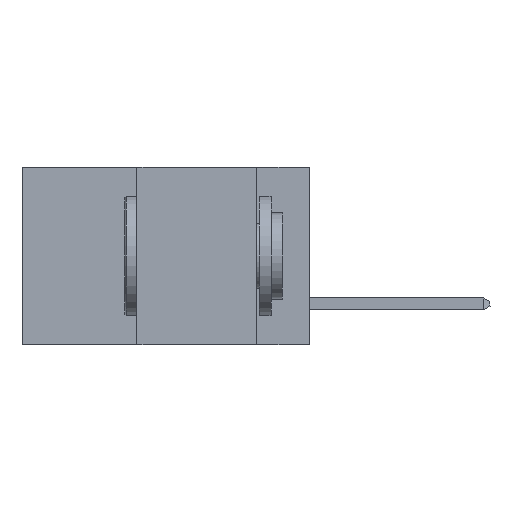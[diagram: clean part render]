
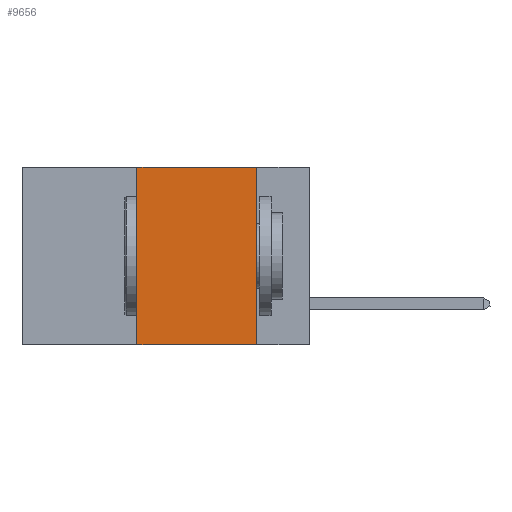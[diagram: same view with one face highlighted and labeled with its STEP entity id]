
A CAD part, left-side view. The second image highlights one B-rep face of the part: STEP entity #9656.
In plain terms, the highlighted planar face has unit normal (-1, 0, 0).
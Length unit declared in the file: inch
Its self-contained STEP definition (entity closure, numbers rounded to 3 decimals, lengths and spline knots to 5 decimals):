
#325 = EDGE_CURVE ( 'NONE', #12321, #18947, #13030, .T. ) ;
#816 = LINE ( 'NONE', #14119, #26722 ) ;
#1361 = CARTESIAN_POINT ( 'NONE',  ( 0., 0.11, -0.37 ) ) ;
#1591 = DIRECTION ( 'NONE',  ( 0., -1., 0. ) ) ;
#4302 = DIRECTION ( 'NONE',  ( 0., -1., 0. ) ) ;
#7045 = VECTOR ( 'NONE', #4302, 39.37008 ) ;
#8223 = PLANE ( 'NONE',  #11939 ) ;
#8604 = CARTESIAN_POINT ( 'NONE',  ( 0., 0.11, 0. ) ) ;
#9656 = ADVANCED_FACE ( 'NONE', ( #30297 ), #8223, .F. ) ;
#10484 = CARTESIAN_POINT ( 'NONE',  ( 0., 0.36, 0. ) ) ;
#10523 = EDGE_CURVE ( 'NONE', #21391, #27044, #12440, .T. ) ;
#11550 = DIRECTION ( 'NONE',  ( 0., 0., -1. ) ) ;
#11801 = CARTESIAN_POINT ( 'NONE',  ( 0., 0.36, -0.37 ) ) ;
#11939 = AXIS2_PLACEMENT_3D ( 'NONE', #28172, #13237, #30655 ) ;
#12262 = VECTOR ( 'NONE', #20417, 39.37008 ) ;
#12321 = VERTEX_POINT ( 'NONE', #11801 ) ;
#12440 = LINE ( 'NONE', #26503, #19905 ) ;
#13030 = LINE ( 'NONE', #25586, #12262 ) ;
#13077 = ORIENTED_EDGE ( 'NONE', *, *, #31139, .T. ) ;
#13237 = DIRECTION ( 'NONE',  ( 1., 0., 0. ) ) ;
#13458 = EDGE_CURVE ( 'NONE', #18947, #21391, #816, .T. ) ;
#14119 = CARTESIAN_POINT ( 'NONE',  ( 0., 0.6, 0. ) ) ;
#15804 = ORIENTED_EDGE ( 'NONE', *, *, #10523, .F. ) ;
#18947 = VERTEX_POINT ( 'NONE', #10484 ) ;
#19905 = VECTOR ( 'NONE', #11550, 39.37008 ) ;
#20417 = DIRECTION ( 'NONE',  ( 0., 0., 1. ) ) ;
#21391 = VERTEX_POINT ( 'NONE', #8604 ) ;
#23134 = EDGE_LOOP ( 'NONE', ( #15804, #29039, #32108, #13077 ) ) ;
#24305 = CARTESIAN_POINT ( 'NONE',  ( 0., 0.6, -0.37 ) ) ;
#25586 = CARTESIAN_POINT ( 'NONE',  ( 0., 0.36, 0. ) ) ;
#26203 = LINE ( 'NONE', #24305, #7045 ) ;
#26503 = CARTESIAN_POINT ( 'NONE',  ( 0., 0.11, 0. ) ) ;
#26722 = VECTOR ( 'NONE', #1591, 39.37008 ) ;
#27044 = VERTEX_POINT ( 'NONE', #1361 ) ;
#28172 = CARTESIAN_POINT ( 'NONE',  ( 0., 0.6, 0. ) ) ;
#29039 = ORIENTED_EDGE ( 'NONE', *, *, #13458, .F. ) ;
#30297 = FACE_OUTER_BOUND ( 'NONE', #23134, .T. ) ;
#30655 = DIRECTION ( 'NONE',  ( 0., 0., -1. ) ) ;
#31139 = EDGE_CURVE ( 'NONE', #12321, #27044, #26203, .T. ) ;
#32108 = ORIENTED_EDGE ( 'NONE', *, *, #325, .F. ) ;
